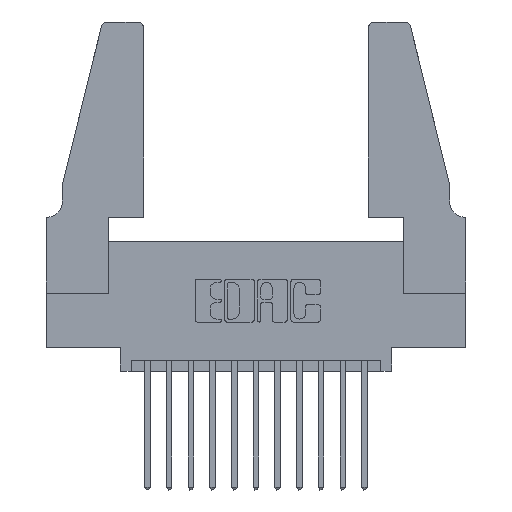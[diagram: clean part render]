
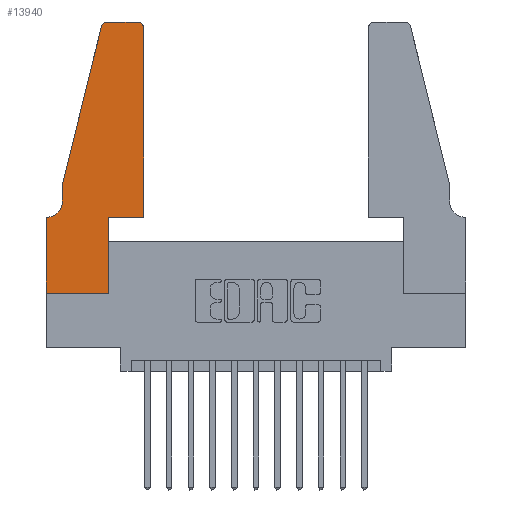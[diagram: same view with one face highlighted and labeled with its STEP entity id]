
A CAD part, top view. The second image highlights one B-rep face of the part: STEP entity #13940.
In plain terms, the highlighted planar face has unit normal (0, 0, 1).
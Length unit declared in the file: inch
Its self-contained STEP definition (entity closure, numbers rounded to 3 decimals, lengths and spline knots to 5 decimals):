
#125 = DIRECTION ( 'NONE',  ( -1., 0., 0. ) ) ;
#212 = CARTESIAN_POINT ( 'NONE',  ( 0.0055, 0.35, 0.37 ) ) ;
#594 = VERTEX_POINT ( 'NONE', #14089 ) ;
#631 = LINE ( 'NONE', #11843, #6637 ) ;
#711 = DIRECTION ( 'NONE',  ( 1., 0., 0. ) ) ;
#790 = VERTEX_POINT ( 'NONE', #2083 ) ;
#819 = EDGE_CURVE ( 'NONE', #7184, #1793, #5006, .T. ) ;
#954 = EDGE_CURVE ( 'NONE', #790, #8383, #631, .T. ) ;
#968 = VERTEX_POINT ( 'NONE', #9499 ) ;
#1099 = ORIENTED_EDGE ( 'NONE', *, *, #9618, .T. ) ;
#1176 = VECTOR ( 'NONE', #9182, 39.37008 ) ;
#1594 = EDGE_CURVE ( 'NONE', #8383, #14103, #6436, .T. ) ;
#1601 = AXIS2_PLACEMENT_3D ( 'NONE', #14694, #1866, #711 ) ;
#1689 = ORIENTED_EDGE ( 'NONE', *, *, #12987, .T. ) ;
#1793 = VERTEX_POINT ( 'NONE', #3853 ) ;
#1866 = DIRECTION ( 'NONE',  ( 0., 0., 1. ) ) ;
#2083 = CARTESIAN_POINT ( 'NONE',  ( 0.0755, 0.5, 0.37 ) ) ;
#2106 = VECTOR ( 'NONE', #8568, 39.37008 ) ;
#2479 = DIRECTION ( 'NONE',  ( 1., 0., 0. ) ) ;
#2895 = ORIENTED_EDGE ( 'NONE', *, *, #6909, .T. ) ;
#2900 = AXIS2_PLACEMENT_3D ( 'NONE', #11457, #4442, #5611 ) ;
#2909 = CIRCLE ( 'NONE', #1601, 0.03 ) ;
#2942 = CARTESIAN_POINT ( 'NONE',  ( 0., 0., 0.37 ) ) ;
#3272 = DIRECTION ( 'NONE',  ( 0., 1., 0. ) ) ;
#3526 = VECTOR ( 'NONE', #125, 39.37008 ) ;
#3768 = VECTOR ( 'NONE', #3272, 39.37008 ) ;
#3792 = EDGE_CURVE ( 'NONE', #1793, #5416, #14293, .T. ) ;
#3853 = CARTESIAN_POINT ( 'NONE',  ( 0.2865, 0., 0.37 ) ) ;
#4060 = LINE ( 'NONE', #14127, #3526 ) ;
#4269 = LINE ( 'NONE', #8237, #9218 ) ;
#4442 = DIRECTION ( 'NONE',  ( 0., 0., 1. ) ) ;
#4513 = CARTESIAN_POINT ( 'NONE',  ( 0., 0.35, 0.37 ) ) ;
#4567 = EDGE_CURVE ( 'NONE', #11591, #7184, #8936, .T. ) ;
#4660 = EDGE_CURVE ( 'NONE', #10150, #8213, #2909, .T. ) ;
#4888 = DIRECTION ( 'NONE',  ( 0., -1., 0. ) ) ;
#4963 = LINE ( 'NONE', #8041, #12630 ) ;
#5006 = LINE ( 'NONE', #10264, #1176 ) ;
#5042 = CARTESIAN_POINT ( 'NONE',  ( 0.2605, 1.25, 0.37 ) ) ;
#5258 = CARTESIAN_POINT ( 'NONE',  ( 0.4505, 0.35, 0.37 ) ) ;
#5416 = VERTEX_POINT ( 'NONE', #13676 ) ;
#5611 = DIRECTION ( 'NONE',  ( 1., 0., 0. ) ) ;
#5962 = ORIENTED_EDGE ( 'NONE', *, *, #6564, .T. ) ;
#5980 = ORIENTED_EDGE ( 'NONE', *, *, #1594, .T. ) ;
#6014 = DIRECTION ( 'NONE',  ( 0., 1., 0. ) ) ;
#6025 = VERTEX_POINT ( 'NONE', #5258 ) ;
#6436 = CIRCLE ( 'NONE', #12095, 0.07 ) ;
#6558 = VECTOR ( 'NONE', #12130, 39.37008 ) ;
#6564 = EDGE_CURVE ( 'NONE', #968, #10150, #9608, .T. ) ;
#6637 = VECTOR ( 'NONE', #4888, 39.37008 ) ;
#6761 = VECTOR ( 'NONE', #6014, 39.37008 ) ;
#6909 = EDGE_CURVE ( 'NONE', #594, #968, #7032, .T. ) ;
#7032 = CIRCLE ( 'NONE', #2900, 0.03 ) ;
#7172 = ORIENTED_EDGE ( 'NONE', *, *, #954, .T. ) ;
#7184 = VERTEX_POINT ( 'NONE', #10847 ) ;
#7199 = ORIENTED_EDGE ( 'NONE', *, *, #819, .T. ) ;
#7335 = ORIENTED_EDGE ( 'NONE', *, *, #3792, .T. ) ;
#7924 = CARTESIAN_POINT ( 'NONE',  ( 0.25487, 1.22718, 0.37 ) ) ;
#8041 = CARTESIAN_POINT ( 'NONE',  ( 0.4505, 0.35, 0.37 ) ) ;
#8213 = VERTEX_POINT ( 'NONE', #7924 ) ;
#8230 = DIRECTION ( 'NONE',  ( -1., 0., 0. ) ) ;
#8237 = CARTESIAN_POINT ( 'NONE',  ( 0.0755, 0.5, 0.37 ) ) ;
#8283 = CARTESIAN_POINT ( 'NONE',  ( 0.0755, 0.42, 0.37 ) ) ;
#8383 = VERTEX_POINT ( 'NONE', #8283 ) ;
#8568 = DIRECTION ( 'NONE',  ( -1., 0., 0. ) ) ;
#8936 = LINE ( 'NONE', #2942, #6558 ) ;
#9030 = EDGE_CURVE ( 'NONE', #14103, #11591, #4060, .T. ) ;
#9182 = DIRECTION ( 'NONE',  ( 1., 0., 0. ) ) ;
#9218 = VECTOR ( 'NONE', #10569, 39.37008 ) ;
#9435 = PLANE ( 'NONE',  #14299 ) ;
#9499 = CARTESIAN_POINT ( 'NONE',  ( 0.4205, 1.25, 0.37 ) ) ;
#9608 = LINE ( 'NONE', #5042, #2106 ) ;
#9618 = EDGE_CURVE ( 'NONE', #5416, #6025, #4963, .T. ) ;
#9716 = ORIENTED_EDGE ( 'NONE', *, *, #9030, .T. ) ;
#9738 = ORIENTED_EDGE ( 'NONE', *, *, #4567, .T. ) ;
#9813 = ORIENTED_EDGE ( 'NONE', *, *, #4660, .T. ) ;
#9949 = FACE_OUTER_BOUND ( 'NONE', #11224, .T. ) ;
#9980 = LINE ( 'NONE', #14525, #3768 ) ;
#10150 = VERTEX_POINT ( 'NONE', #12772 ) ;
#10264 = CARTESIAN_POINT ( 'NONE',  ( 0., 0., 0.37 ) ) ;
#10305 = DIRECTION ( 'NONE',  ( 1., 0., 0. ) ) ;
#10460 = CARTESIAN_POINT ( 'NONE',  ( 0., 0.35, 0.37 ) ) ;
#10569 = DIRECTION ( 'NONE',  ( -0.239, -0.971, 0. ) ) ;
#10616 = DIRECTION ( 'NONE',  ( 0., 0., 1. ) ) ;
#10660 = DIRECTION ( 'NONE',  ( 0., 0., -1. ) ) ;
#10787 = CARTESIAN_POINT ( 'NONE',  ( 0.2865, 0.35, 0.37 ) ) ;
#10847 = CARTESIAN_POINT ( 'NONE',  ( 0., 0., 0.37 ) ) ;
#11224 = EDGE_LOOP ( 'NONE', ( #5962, #9813, #12389, #7172, #5980, #9716, #9738, #7199, #7335, #1099, #1689, #2895 ) ) ;
#11457 = CARTESIAN_POINT ( 'NONE',  ( 0.4205, 1.22, 0.37 ) ) ;
#11591 = VERTEX_POINT ( 'NONE', #4513 ) ;
#11843 = CARTESIAN_POINT ( 'NONE',  ( 0.0755, 0.5, 0.37 ) ) ;
#12095 = AXIS2_PLACEMENT_3D ( 'NONE', #12959, #10660, #8230 ) ;
#12130 = DIRECTION ( 'NONE',  ( 0., -1., 0. ) ) ;
#12389 = ORIENTED_EDGE ( 'NONE', *, *, #13879, .T. ) ;
#12630 = VECTOR ( 'NONE', #10305, 39.37008 ) ;
#12772 = CARTESIAN_POINT ( 'NONE',  ( 0.284, 1.25, 0.37 ) ) ;
#12959 = CARTESIAN_POINT ( 'NONE',  ( 0.0055, 0.42, 0.37 ) ) ;
#12987 = EDGE_CURVE ( 'NONE', #6025, #594, #9980, .T. ) ;
#13676 = CARTESIAN_POINT ( 'NONE',  ( 0.2865, 0.35, 0.37 ) ) ;
#13879 = EDGE_CURVE ( 'NONE', #8213, #790, #4269, .T. ) ;
#13940 = ADVANCED_FACE ( 'NONE', ( #9949 ), #9435, .T. ) ;
#14089 = CARTESIAN_POINT ( 'NONE',  ( 0.4505, 1.22, 0.37 ) ) ;
#14103 = VERTEX_POINT ( 'NONE', #212 ) ;
#14127 = CARTESIAN_POINT ( 'NONE',  ( 0.0755, 0.35, 0.37 ) ) ;
#14293 = LINE ( 'NONE', #10787, #6761 ) ;
#14299 = AXIS2_PLACEMENT_3D ( 'NONE', #10460, #10616, #2479 ) ;
#14525 = CARTESIAN_POINT ( 'NONE',  ( 0.4505, 0.35, 0.37 ) ) ;
#14694 = CARTESIAN_POINT ( 'NONE',  ( 0.284, 1.22, 0.37 ) ) ;
